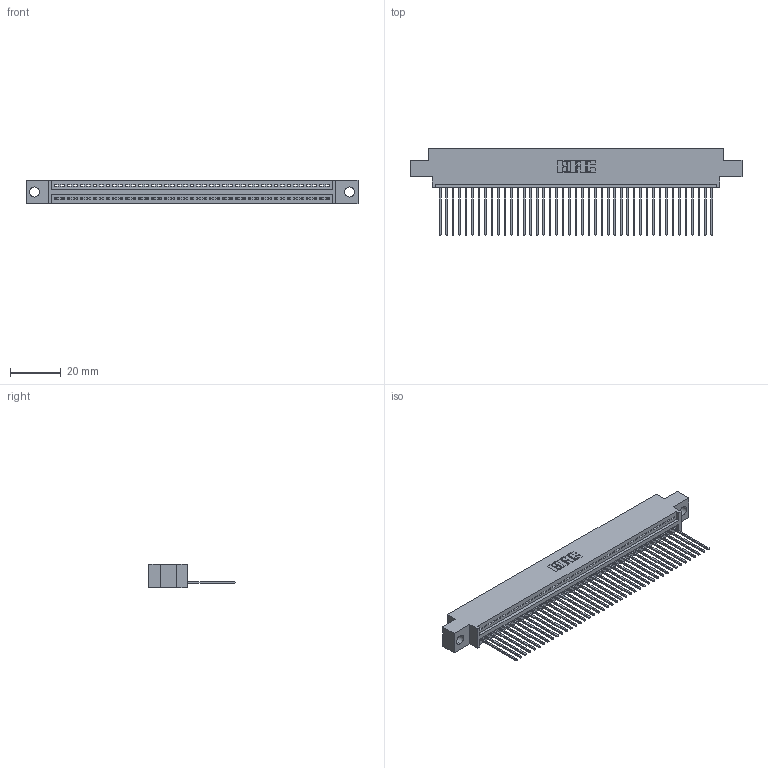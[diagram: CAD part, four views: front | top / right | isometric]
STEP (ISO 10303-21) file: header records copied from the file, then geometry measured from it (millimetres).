
FILE_DESCRIPTION (( 'STEP AP203' ), '1' );
FILE_NAME ('345-043-541-604.STEP', '2021-05-26T15:04:56', ( '' ), ( '' ), 'SwSTEP 2.0', 'SolidWorks 2020', '' );
FILE_SCHEMA (( 'CONFIG_CONTROL_DESIGN' ));
Length unit declared in the file: inch
Products named in the file (3): 345-043-541-604; 345 Part_0.170 Offset - 0.156 Dia-TI; 345-292-001_345-293-141
Assembly tree (44 placements, depth 2):
  345-043-541-604
    345 Part_0.170 Offset - 0.156 Dia-TI
    345-292-001_345-293-141  x43
Bounding box: 130.43 x 33.96 x 9.4 mm (x, y, z)
Volume: 12319 mm3; surface area: 17188.4 mm2
Topology: 44 solids, 44 shells, 2638 faces, 7957 edges, 5246 vertices
Faces by surface type: plane 1818, cylinder 820
Entity records: 32797 total; most frequent: CARTESIAN_POINT 5691, ORIENTED_EDGE 5666, DIRECTION 4967, EDGE_CURVE 2833, LINE 2529, VECTOR 2529, VERTEX_POINT 1886, AXIS2_PLACEMENT_3D 1219
